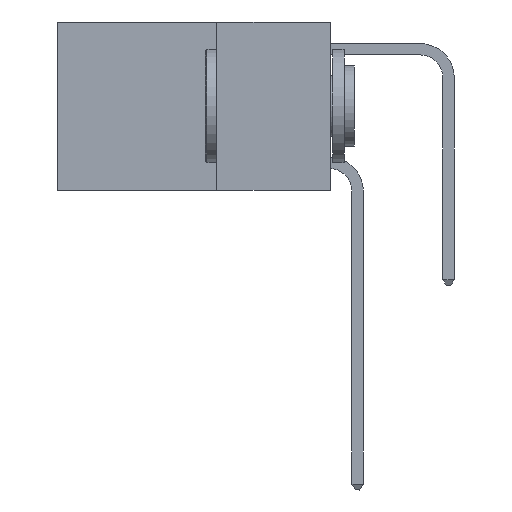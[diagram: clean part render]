
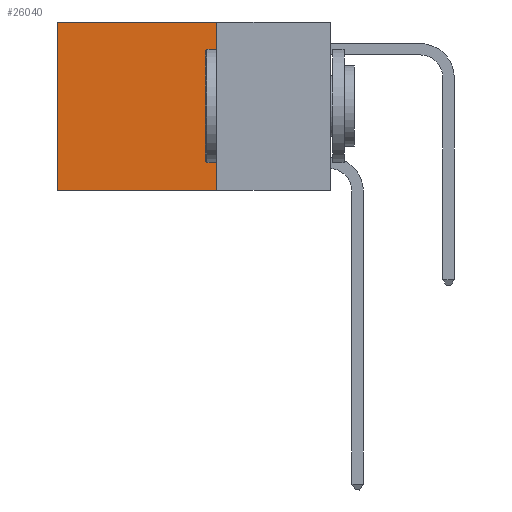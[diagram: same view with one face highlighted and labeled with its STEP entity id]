
A CAD part, left-side view. The second image highlights one B-rep face of the part: STEP entity #26040.
In plain terms, the highlighted planar face has unit normal (-1, 0, 0).
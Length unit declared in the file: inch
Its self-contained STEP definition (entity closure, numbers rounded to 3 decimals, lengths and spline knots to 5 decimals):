
#115 = LINE ( 'NONE', #4552, #15156 ) ;
#429 = CARTESIAN_POINT ( 'NONE',  ( 0.2625, 0.25, 0. ) ) ;
#2171 = CARTESIAN_POINT ( 'NONE',  ( 0.2625, 0.25, 0. ) ) ;
#2721 = DIRECTION ( 'NONE',  ( 0., 0., -1. ) ) ;
#3574 = LINE ( 'NONE', #8159, #24965 ) ;
#4068 = CARTESIAN_POINT ( 'NONE',  ( 0.2625, 0.6, 0. ) ) ;
#4552 = CARTESIAN_POINT ( 'NONE',  ( 0.2625, 0.25, 0. ) ) ;
#6872 = PLANE ( 'NONE',  #8280 ) ;
#8120 = VERTEX_POINT ( 'NONE', #21159 ) ;
#8159 = CARTESIAN_POINT ( 'NONE',  ( 0.2625, 0.25, -0.37 ) ) ;
#8280 = AXIS2_PLACEMENT_3D ( 'NONE', #429, #26065, #13934 ) ;
#8330 = ORIENTED_EDGE ( 'NONE', *, *, #13693, .F. ) ;
#10249 = VECTOR ( 'NONE', #27967, 39.37008 ) ;
#10670 = LINE ( 'NONE', #4068, #15107 ) ;
#12105 = VERTEX_POINT ( 'NONE', #21900 ) ;
#12728 = EDGE_CURVE ( 'NONE', #8120, #21967, #10670, .T. ) ;
#12803 = VERTEX_POINT ( 'NONE', #13587 ) ;
#12982 = ORIENTED_EDGE ( 'NONE', *, *, #12728, .T. ) ;
#13587 = CARTESIAN_POINT ( 'NONE',  ( 0.2625, 0.25, 0. ) ) ;
#13693 = EDGE_CURVE ( 'NONE', #12803, #12105, #115, .T. ) ;
#13934 = DIRECTION ( 'NONE',  ( 0., 0., -1. ) ) ;
#15107 = VECTOR ( 'NONE', #18018, 39.37008 ) ;
#15156 = VECTOR ( 'NONE', #2721, 39.37008 ) ;
#16069 = ORIENTED_EDGE ( 'NONE', *, *, #28275, .T. ) ;
#16257 = CARTESIAN_POINT ( 'NONE',  ( 0.2625, 0.6, -0.37 ) ) ;
#16678 = FACE_OUTER_BOUND ( 'NONE', #22489, .T. ) ;
#18018 = DIRECTION ( 'NONE',  ( 0., 0., -1. ) ) ;
#18989 = ORIENTED_EDGE ( 'NONE', *, *, #27305, .F. ) ;
#20414 = LINE ( 'NONE', #2171, #10249 ) ;
#21159 = CARTESIAN_POINT ( 'NONE',  ( 0.2625, 0.6, 0. ) ) ;
#21900 = CARTESIAN_POINT ( 'NONE',  ( 0.2625, 0.25, -0.37 ) ) ;
#21967 = VERTEX_POINT ( 'NONE', #16257 ) ;
#22489 = EDGE_LOOP ( 'NONE', ( #12982, #18989, #8330, #16069 ) ) ;
#24900 = DIRECTION ( 'NONE',  ( 0., 1., 0. ) ) ;
#24965 = VECTOR ( 'NONE', #24900, 39.37008 ) ;
#26040 = ADVANCED_FACE ( 'NONE', ( #16678 ), #6872, .F. ) ;
#26065 = DIRECTION ( 'NONE',  ( 1., 0., 0. ) ) ;
#27305 = EDGE_CURVE ( 'NONE', #12105, #21967, #3574, .T. ) ;
#27967 = DIRECTION ( 'NONE',  ( 0., 1., 0. ) ) ;
#28275 = EDGE_CURVE ( 'NONE', #12803, #8120, #20414, .T. ) ;
